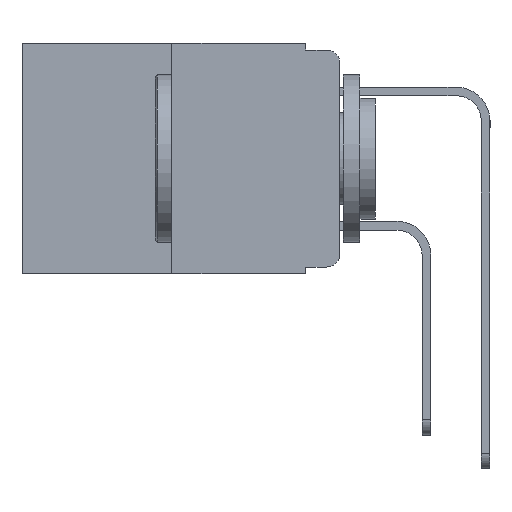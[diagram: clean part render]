
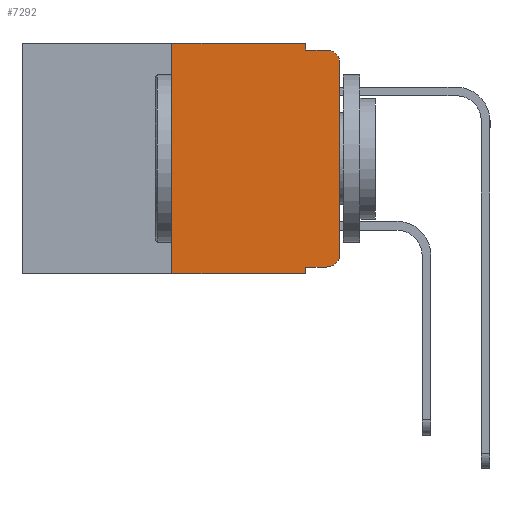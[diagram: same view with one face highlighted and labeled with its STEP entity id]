
A CAD part, left-side view. The second image highlights one B-rep face of the part: STEP entity #7292.
In plain terms, the highlighted planar face has unit normal (-1, 0, 0).
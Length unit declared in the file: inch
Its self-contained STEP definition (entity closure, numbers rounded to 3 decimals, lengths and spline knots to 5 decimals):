
#410 = LINE ( 'NONE', #4106, #4228 ) ;
#644 = ORIENTED_EDGE ( 'NONE', *, *, #10286, .T. ) ;
#773 = VERTEX_POINT ( 'NONE', #12921 ) ;
#988 = DIRECTION ( 'NONE',  ( 0., 0., -1. ) ) ;
#1602 = CARTESIAN_POINT ( 'NONE',  ( 0., 0.02, -0.03 ) ) ;
#1702 = DIRECTION ( 'NONE',  ( 0., -1., 0. ) ) ;
#1909 = ORIENTED_EDGE ( 'NONE', *, *, #10305, .T. ) ;
#2129 = VERTEX_POINT ( 'NONE', #14732 ) ;
#2385 = VERTEX_POINT ( 'NONE', #14359 ) ;
#2469 = CARTESIAN_POINT ( 'NONE',  ( 0., 0.473, -0.343 ) ) ;
#2506 = ORIENTED_EDGE ( 'NONE', *, *, #10242, .T. ) ;
#2668 = EDGE_CURVE ( 'NONE', #3289, #5993, #10450, .T. ) ;
#2877 = DIRECTION ( 'NONE',  ( 0., 0., -1. ) ) ;
#3289 = VERTEX_POINT ( 'NONE', #7294 ) ;
#3677 = ORIENTED_EDGE ( 'NONE', *, *, #7403, .T. ) ;
#3837 = CIRCLE ( 'NONE', #13396, 0.02 ) ;
#4106 = CARTESIAN_POINT ( 'NONE',  ( 0., 0.051, -0.01 ) ) ;
#4203 = AXIS2_PLACEMENT_3D ( 'NONE', #13947, #6798, #15108 ) ;
#4218 = CARTESIAN_POINT ( 'NONE',  ( 0., 0.051, -0.333 ) ) ;
#4228 = VECTOR ( 'NONE', #14904, 39.37008 ) ;
#4386 = VECTOR ( 'NONE', #6475, 39.37008 ) ;
#4936 = DIRECTION ( 'NONE',  ( 0., -1., 0. ) ) ;
#5172 = CIRCLE ( 'NONE', #4203, 0.02 ) ;
#5966 = VECTOR ( 'NONE', #15010, 39.37008 ) ;
#5993 = VERTEX_POINT ( 'NONE', #8397 ) ;
#6030 = VECTOR ( 'NONE', #4936, 39.37008 ) ;
#6475 = DIRECTION ( 'NONE',  ( 0., -1., 0. ) ) ;
#6524 = DIRECTION ( 'NONE',  ( 0., 0., 1. ) ) ;
#6581 = CARTESIAN_POINT ( 'NONE',  ( 0., 0.051, 0. ) ) ;
#6640 = DIRECTION ( 'NONE',  ( 0., 0., 1. ) ) ;
#6690 = CARTESIAN_POINT ( 'NONE',  ( 0., 0.051, 0. ) ) ;
#6730 = LINE ( 'NONE', #6581, #13832 ) ;
#6798 = DIRECTION ( 'NONE',  ( -1., 0., 0. ) ) ;
#6948 = CARTESIAN_POINT ( 'NONE',  ( 0., 0.051, -0.343 ) ) ;
#6950 = AXIS2_PLACEMENT_3D ( 'NONE', #14315, #8412, #988 ) ;
#7071 = CARTESIAN_POINT ( 'NONE',  ( 0., 0.473, 0. ) ) ;
#7292 = ADVANCED_FACE ( 'NONE', ( #10741 ), #15488, .F. ) ;
#7294 = CARTESIAN_POINT ( 'NONE',  ( 0., 0.25, 0. ) ) ;
#7403 = EDGE_CURVE ( 'NONE', #15301, #10360, #12397, .T. ) ;
#7817 = DIRECTION ( 'NONE',  ( 0., 0., -1. ) ) ;
#8397 = CARTESIAN_POINT ( 'NONE',  ( 0., 0.051, 0. ) ) ;
#8412 = DIRECTION ( 'NONE',  ( 1., 0., 0. ) ) ;
#8805 = VECTOR ( 'NONE', #1702, 39.37008 ) ;
#9171 = LINE ( 'NONE', #6690, #5966 ) ;
#9208 = CARTESIAN_POINT ( 'NONE',  ( 0., 0.25, -0.343 ) ) ;
#9428 = VERTEX_POINT ( 'NONE', #11094 ) ;
#9544 = LINE ( 'NONE', #13800, #15821 ) ;
#10130 = ORIENTED_EDGE ( 'NONE', *, *, #10284, .F. ) ;
#10158 = DIRECTION ( 'NONE',  ( -1., 0., 0. ) ) ;
#10242 = EDGE_CURVE ( 'NONE', #10259, #2129, #10681, .T. ) ;
#10243 = EDGE_CURVE ( 'NONE', #2129, #773, #3837, .T. ) ;
#10259 = VERTEX_POINT ( 'NONE', #13758 ) ;
#10261 = EDGE_CURVE ( 'NONE', #13325, #773, #410, .T. ) ;
#10263 = EDGE_CURVE ( 'NONE', #5993, #13325, #6730, .T. ) ;
#10266 = EDGE_CURVE ( 'NONE', #15301, #3289, #9544, .T. ) ;
#10284 = EDGE_CURVE ( 'NONE', #9428, #10360, #9171, .T. ) ;
#10286 = EDGE_CURVE ( 'NONE', #9428, #2385, #15465, .T. ) ;
#10305 = EDGE_CURVE ( 'NONE', #2385, #10259, #5172, .T. ) ;
#10306 = VECTOR ( 'NONE', #6524, 39.37008 ) ;
#10360 = VERTEX_POINT ( 'NONE', #6948 ) ;
#10450 = LINE ( 'NONE', #7071, #4386 ) ;
#10496 = ORIENTED_EDGE ( 'NONE', *, *, #10243, .T. ) ;
#10681 = LINE ( 'NONE', #12490, #10306 ) ;
#10741 = FACE_OUTER_BOUND ( 'NONE', #14827, .T. ) ;
#11094 = CARTESIAN_POINT ( 'NONE',  ( 0., 0.051, -0.333 ) ) ;
#12063 = CARTESIAN_POINT ( 'NONE',  ( 0., 0.051, -0.01 ) ) ;
#12397 = LINE ( 'NONE', #2469, #6030 ) ;
#12490 = CARTESIAN_POINT ( 'NONE',  ( 0., 0., 0. ) ) ;
#12531 = ORIENTED_EDGE ( 'NONE', *, *, #2668, .F. ) ;
#12710 = ORIENTED_EDGE ( 'NONE', *, *, #10261, .F. ) ;
#12921 = CARTESIAN_POINT ( 'NONE',  ( 0., 0.02, -0.01 ) ) ;
#13325 = VERTEX_POINT ( 'NONE', #12063 ) ;
#13396 = AXIS2_PLACEMENT_3D ( 'NONE', #1602, #10158, #2877 ) ;
#13758 = CARTESIAN_POINT ( 'NONE',  ( 0., 0., -0.313 ) ) ;
#13800 = CARTESIAN_POINT ( 'NONE',  ( 0., 0.25, 0. ) ) ;
#13832 = VECTOR ( 'NONE', #7817, 39.37008 ) ;
#13846 = ORIENTED_EDGE ( 'NONE', *, *, #10263, .F. ) ;
#13947 = CARTESIAN_POINT ( 'NONE',  ( 0., 0.02, -0.313 ) ) ;
#14315 = CARTESIAN_POINT ( 'NONE',  ( 0., 0.473, 0. ) ) ;
#14359 = CARTESIAN_POINT ( 'NONE',  ( 0., 0.02, -0.333 ) ) ;
#14732 = CARTESIAN_POINT ( 'NONE',  ( 0., 0., -0.03 ) ) ;
#14827 = EDGE_LOOP ( 'NONE', ( #2506, #10496, #12710, #13846, #12531, #15673, #3677, #10130, #644, #1909 ) ) ;
#14904 = DIRECTION ( 'NONE',  ( 0., -1., 0. ) ) ;
#15010 = DIRECTION ( 'NONE',  ( 0., 0., -1. ) ) ;
#15108 = DIRECTION ( 'NONE',  ( 0., 0., -1. ) ) ;
#15301 = VERTEX_POINT ( 'NONE', #9208 ) ;
#15465 = LINE ( 'NONE', #4218, #8805 ) ;
#15488 = PLANE ( 'NONE',  #6950 ) ;
#15673 = ORIENTED_EDGE ( 'NONE', *, *, #10266, .F. ) ;
#15821 = VECTOR ( 'NONE', #6640, 39.37008 ) ;
